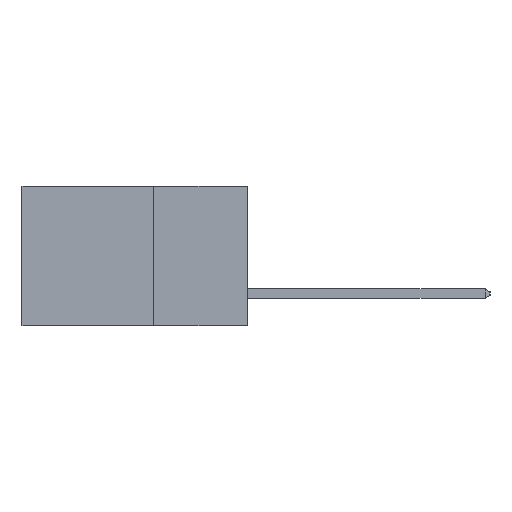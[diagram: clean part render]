
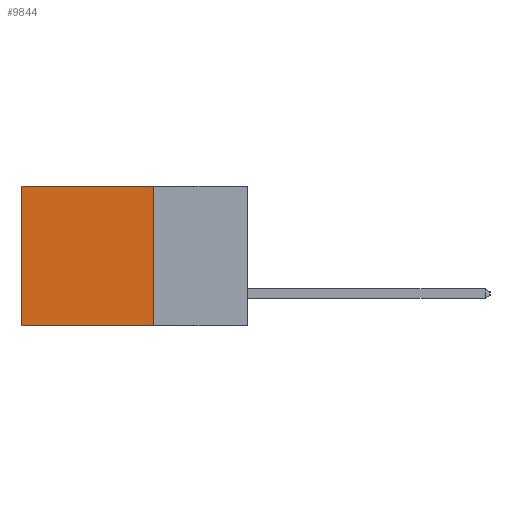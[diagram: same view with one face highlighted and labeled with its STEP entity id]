
A CAD part, left-side view. The second image highlights one B-rep face of the part: STEP entity #9844.
In plain terms, the highlighted planar face has unit normal (-1, 0, 0).
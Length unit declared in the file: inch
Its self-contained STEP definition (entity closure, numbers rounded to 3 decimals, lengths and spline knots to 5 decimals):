
#376 = CARTESIAN_POINT ( 'NONE',  ( 0.298, 0.25, -0.37 ) ) ;
#506 = EDGE_CURVE ( 'NONE', #5529, #1494, #3792, .T. ) ;
#1284 = DIRECTION ( 'NONE',  ( 0., 1., 0. ) ) ;
#1373 = VERTEX_POINT ( 'NONE', #8660 ) ;
#1494 = VERTEX_POINT ( 'NONE', #8504 ) ;
#1900 = FACE_OUTER_BOUND ( 'NONE', #11054, .T. ) ;
#1969 = LINE ( 'NONE', #3573, #11105 ) ;
#2030 = CARTESIAN_POINT ( 'NONE',  ( 0.298, 0.25, 0. ) ) ;
#2211 = CARTESIAN_POINT ( 'NONE',  ( 0.298, 0.6, 0. ) ) ;
#2479 = EDGE_CURVE ( 'NONE', #5529, #9783, #1969, .T. ) ;
#3227 = DIRECTION ( 'NONE',  ( 0., 0., -1. ) ) ;
#3252 = ORIENTED_EDGE ( 'NONE', *, *, #2479, .T. ) ;
#3292 = LINE ( 'NONE', #376, #7724 ) ;
#3573 = CARTESIAN_POINT ( 'NONE',  ( 0.298, 0.25, 0. ) ) ;
#3792 = LINE ( 'NONE', #2030, #10585 ) ;
#4456 = DIRECTION ( 'NONE',  ( 0., 1., 0. ) ) ;
#4792 = CARTESIAN_POINT ( 'NONE',  ( 0.298, 0.25, 0. ) ) ;
#4905 = CARTESIAN_POINT ( 'NONE',  ( 0.298, 0.6, 0. ) ) ;
#5529 = VERTEX_POINT ( 'NONE', #4792 ) ;
#5552 = AXIS2_PLACEMENT_3D ( 'NONE', #6716, #8533, #3227 ) ;
#5960 = VECTOR ( 'NONE', #8522, 39.37008 ) ;
#6716 = CARTESIAN_POINT ( 'NONE',  ( 0.298, 0.25, 0. ) ) ;
#6728 = ORIENTED_EDGE ( 'NONE', *, *, #6849, .T. ) ;
#6849 = EDGE_CURVE ( 'NONE', #9783, #1373, #8331, .T. ) ;
#7724 = VECTOR ( 'NONE', #1284, 39.37008 ) ;
#8102 = ORIENTED_EDGE ( 'NONE', *, *, #506, .F. ) ;
#8331 = LINE ( 'NONE', #4905, #5960 ) ;
#8504 = CARTESIAN_POINT ( 'NONE',  ( 0.298, 0.25, -0.37 ) ) ;
#8522 = DIRECTION ( 'NONE',  ( 0., 0., -1. ) ) ;
#8533 = DIRECTION ( 'NONE',  ( 1., 0., 0. ) ) ;
#8660 = CARTESIAN_POINT ( 'NONE',  ( 0.298, 0.6, -0.37 ) ) ;
#8666 = ORIENTED_EDGE ( 'NONE', *, *, #9301, .F. ) ;
#9301 = EDGE_CURVE ( 'NONE', #1494, #1373, #3292, .T. ) ;
#9430 = DIRECTION ( 'NONE',  ( 0., 0., -1. ) ) ;
#9783 = VERTEX_POINT ( 'NONE', #2211 ) ;
#9844 = ADVANCED_FACE ( 'NONE', ( #1900 ), #10244, .F. ) ;
#10244 = PLANE ( 'NONE',  #5552 ) ;
#10585 = VECTOR ( 'NONE', #9430, 39.37008 ) ;
#11054 = EDGE_LOOP ( 'NONE', ( #6728, #8666, #8102, #3252 ) ) ;
#11105 = VECTOR ( 'NONE', #4456, 39.37008 ) ;
